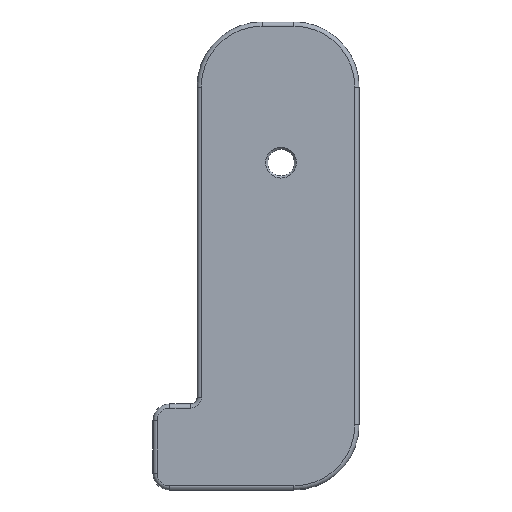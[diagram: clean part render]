
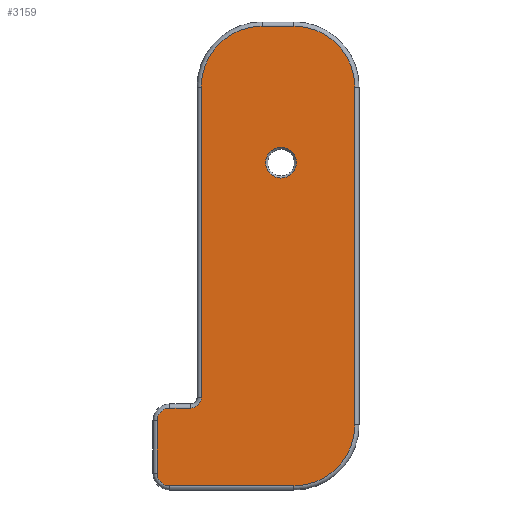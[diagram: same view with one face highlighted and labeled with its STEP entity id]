
A CAD part, front view. The second image highlights one B-rep face of the part: STEP entity #3159.
In plain terms, the highlighted planar face has unit normal (0, -1, 0).
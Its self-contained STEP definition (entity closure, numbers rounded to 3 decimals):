
#54=FACE_BOUND('',#1100,.T.);
#77=PLANE('',#3511);
#283=LINE('',#5519,#549);
#285=LINE('',#5531,#551);
#286=LINE('',#5540,#552);
#288=LINE('',#5552,#554);
#290=LINE('',#5564,#556);
#291=LINE('',#5572,#557);
#549=VECTOR('',#4184,10.);
#551=VECTOR('',#4198,10.);
#552=VECTOR('',#4211,10.);
#554=VECTOR('',#4225,10.);
#556=VECTOR('',#4239,10.);
#557=VECTOR('',#4250,10.);
#883=FACE_OUTER_BOUND('',#1099,.T.);
#1099=EDGE_LOOP('',(#2594,#2595,#2596,#2597,#2598,#2599,#2600,#2601,#2602,
#2603,#2604,#2605));
#1100=EDGE_LOOP('',(#2606));
#1321=CIRCLE('',#3468,1.5);
#1327=CIRCLE('',#3476,1.263);
#1331=CIRCLE('',#3482,7.25);
#1335=CIRCLE('',#3488,7.25);
#1339=CIRCLE('',#3494,7.25);
#1343=CIRCLE('',#3500,1.5);
#1347=CIRCLE('',#3512,1.838);
#1536=VERTEX_POINT('',#5507);
#1537=VERTEX_POINT('',#5509);
#1539=VERTEX_POINT('',#5515);
#1541=VERTEX_POINT('',#5521);
#1543=VERTEX_POINT('',#5527);
#1545=VERTEX_POINT('',#5533);
#1546=VERTEX_POINT('',#5538);
#1547=VERTEX_POINT('',#5542);
#1549=VERTEX_POINT('',#5548);
#1551=VERTEX_POINT('',#5554);
#1553=VERTEX_POINT('',#5560);
#1555=VERTEX_POINT('',#5566);
#1565=VERTEX_POINT('',#5604);
#1885=EDGE_CURVE('',#1536,#1537,#1321,.T.);
#1890=EDGE_CURVE('',#1537,#1539,#283,.T.);
#1893=EDGE_CURVE('',#1539,#1541,#1327,.T.);
#1896=EDGE_CURVE('',#1541,#1543,#285,.T.);
#1899=EDGE_CURVE('',#1543,#1545,#1331,.T.);
#1901=EDGE_CURVE('',#1545,#1546,#286,.T.);
#1904=EDGE_CURVE('',#1546,#1547,#1335,.T.);
#1907=EDGE_CURVE('',#1547,#1549,#288,.T.);
#1910=EDGE_CURVE('',#1549,#1551,#1339,.T.);
#1913=EDGE_CURVE('',#1551,#1553,#290,.T.);
#1916=EDGE_CURVE('',#1553,#1555,#1343,.T.);
#1917=EDGE_CURVE('',#1555,#1536,#291,.T.);
#1934=EDGE_CURVE('',#1565,#1565,#1347,.T.);
#2594=ORIENTED_EDGE('',*,*,#1885,.F.);
#2595=ORIENTED_EDGE('',*,*,#1917,.F.);
#2596=ORIENTED_EDGE('',*,*,#1916,.F.);
#2597=ORIENTED_EDGE('',*,*,#1913,.F.);
#2598=ORIENTED_EDGE('',*,*,#1910,.F.);
#2599=ORIENTED_EDGE('',*,*,#1907,.F.);
#2600=ORIENTED_EDGE('',*,*,#1904,.F.);
#2601=ORIENTED_EDGE('',*,*,#1901,.F.);
#2602=ORIENTED_EDGE('',*,*,#1899,.F.);
#2603=ORIENTED_EDGE('',*,*,#1896,.F.);
#2604=ORIENTED_EDGE('',*,*,#1893,.F.);
#2605=ORIENTED_EDGE('',*,*,#1890,.F.);
#2606=ORIENTED_EDGE('',*,*,#1934,.F.);
#3159=ADVANCED_FACE('',(#883,#54),#77,.T.);
#3468=AXIS2_PLACEMENT_3D('',#5510,#4173,#4174);
#3476=AXIS2_PLACEMENT_3D('',#5525,#4191,#4192);
#3482=AXIS2_PLACEMENT_3D('',#5536,#4205,#4206);
#3488=AXIS2_PLACEMENT_3D('',#5546,#4218,#4219);
#3494=AXIS2_PLACEMENT_3D('',#5558,#4232,#4233);
#3500=AXIS2_PLACEMENT_3D('',#5570,#4246,#4247);
#3511=AXIS2_PLACEMENT_3D('',#5603,#4282,#4283);
#3512=AXIS2_PLACEMENT_3D('',#5605,#4284,#4285);
#4173=DIRECTION('center_axis',(0.,1.,0.));
#4174=DIRECTION('ref_axis',(-0.707,0.,0.707));
#4184=DIRECTION('',(1.,0.,0.));
#4191=DIRECTION('center_axis',(0.,-1.,0.));
#4192=DIRECTION('ref_axis',(0.707,0.,-0.707));
#4198=DIRECTION('',(0.,0.,1.));
#4205=DIRECTION('center_axis',(0.,1.,0.));
#4206=DIRECTION('ref_axis',(-0.707,0.,0.707));
#4211=DIRECTION('',(1.,0.,0.));
#4218=DIRECTION('center_axis',(0.,1.,0.));
#4219=DIRECTION('ref_axis',(0.707,0.,0.707));
#4225=DIRECTION('',(0.,0.,-1.));
#4232=DIRECTION('center_axis',(0.,1.,0.));
#4233=DIRECTION('ref_axis',(0.707,0.,-0.707));
#4239=DIRECTION('',(-1.,0.,0.));
#4246=DIRECTION('center_axis',(0.,1.,0.));
#4247=DIRECTION('ref_axis',(-0.707,0.,-0.707));
#4250=DIRECTION('',(0.,0.,1.));
#4282=DIRECTION('center_axis',(0.,-1.,0.));
#4283=DIRECTION('ref_axis',(1.,0.,0.));
#4284=DIRECTION('center_axis',(0.,-1.,0.));
#4285=DIRECTION('ref_axis',(-1.,0.,0.));
#5507=CARTESIAN_POINT('',(-21.,-2.794,-93.933));
#5509=CARTESIAN_POINT('',(-19.5,-2.794,-92.433));
#5510=CARTESIAN_POINT('Origin',(-19.5,-2.794,-93.933));
#5515=CARTESIAN_POINT('',(-17.013,-2.794,-92.433));
#5519=CARTESIAN_POINT('',(-13.12,-2.794,-92.433));
#5521=CARTESIAN_POINT('',(-15.75,-2.794,-91.171));
#5525=CARTESIAN_POINT('Origin',(-17.013,-2.794,-91.171));
#5527=CARTESIAN_POINT('',(-15.75,-2.794,-54.183));
#5531=CARTESIAN_POINT('',(-15.75,-2.794,-64.246));
#5533=CARTESIAN_POINT('',(-8.5,-2.794,-46.933));
#5536=CARTESIAN_POINT('Origin',(-8.5,-2.794,-54.183));
#5538=CARTESIAN_POINT('',(-4.705,-2.794,-46.933));
#5540=CARTESIAN_POINT('',(-3.091,-2.794,-46.933));
#5542=CARTESIAN_POINT('',(2.545,-2.794,-54.183));
#5546=CARTESIAN_POINT('Origin',(-4.705,-2.794,-54.183));
#5548=CARTESIAN_POINT('',(2.545,-2.794,-94.433));
#5552=CARTESIAN_POINT('',(2.545,-2.794,-88.246));
#5554=CARTESIAN_POINT('',(-4.705,-2.794,-101.683));
#5558=CARTESIAN_POINT('Origin',(-4.705,-2.794,-94.433));
#5560=CARTESIAN_POINT('',(-19.5,-2.794,-101.683));
#5564=CARTESIAN_POINT('',(-15.364,-2.794,-101.683));
#5566=CARTESIAN_POINT('',(-21.,-2.794,-100.183));
#5570=CARTESIAN_POINT('Origin',(-19.5,-2.794,-100.183));
#5572=CARTESIAN_POINT('',(-21.,-2.794,-83.121));
#5603=CARTESIAN_POINT('Origin',(-9.227,-2.794,-74.308));
#5604=CARTESIAN_POINT('',(-4.413,-2.794,-63.183));
#5605=CARTESIAN_POINT('Origin',(-6.25,-2.794,-63.183));
